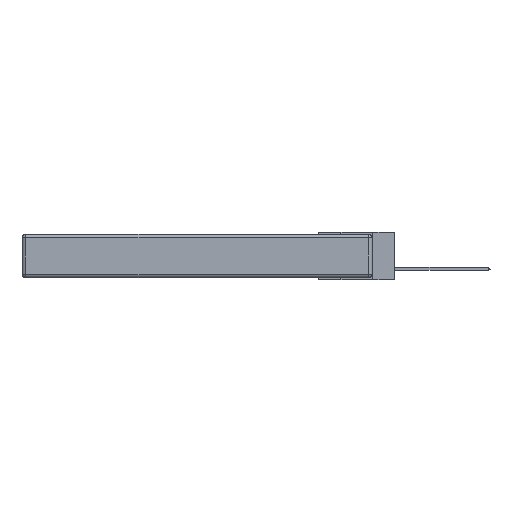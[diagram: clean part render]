
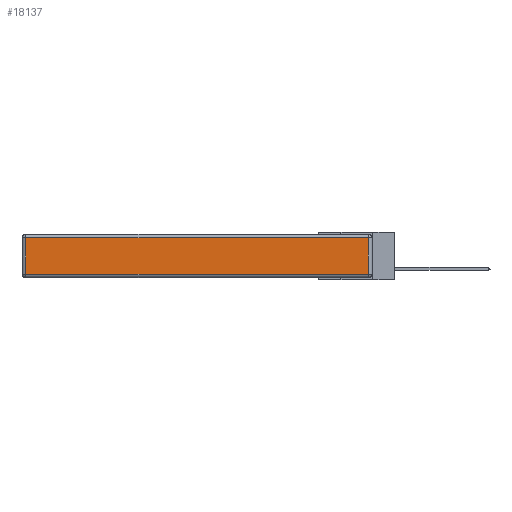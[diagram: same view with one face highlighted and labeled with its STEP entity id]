
A CAD part, left-side view. The second image highlights one B-rep face of the part: STEP entity #18137.
In plain terms, the highlighted planar face has unit normal (-1, 0, 0).
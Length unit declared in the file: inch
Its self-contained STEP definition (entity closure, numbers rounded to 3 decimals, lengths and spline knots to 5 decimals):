
#7 = DIRECTION ( 'NONE',  ( -1., 0., 0. ) ) ;
#1589 = CARTESIAN_POINT ( 'NONE',  ( 0., 2.72, -0.03 ) ) ;
#1965 = CARTESIAN_POINT ( 'NONE',  ( 0., 0.03, -0.343 ) ) ;
#2236 = CARTESIAN_POINT ( 'NONE',  ( 0., 0., -0.343 ) ) ;
#4499 = ORIENTED_EDGE ( 'NONE', *, *, #5396, .T. ) ;
#4649 = EDGE_LOOP ( 'NONE', ( #9485, #4499, #24535, #13601 ) ) ;
#5396 = EDGE_CURVE ( 'NONE', #16382, #19839, #21255, .T. ) ;
#5569 = DIRECTION ( 'NONE',  ( 0., 0., -1. ) ) ;
#6389 = AXIS2_PLACEMENT_3D ( 'NONE', #2236, #7, #12685 ) ;
#6978 = EDGE_CURVE ( 'NONE', #19839, #25002, #9342, .T. ) ;
#8350 = VECTOR ( 'NONE', #25428, 39.37008 ) ;
#8665 = DIRECTION ( 'NONE',  ( 0., 1., 0. ) ) ;
#9079 = LINE ( 'NONE', #18195, #26648 ) ;
#9342 = LINE ( 'NONE', #13171, #26913 ) ;
#9485 = ORIENTED_EDGE ( 'NONE', *, *, #14847, .T. ) ;
#12685 = DIRECTION ( 'NONE',  ( 0., 0., 1. ) ) ;
#13171 = CARTESIAN_POINT ( 'NONE',  ( 0., 2.75, -0.03 ) ) ;
#13601 = ORIENTED_EDGE ( 'NONE', *, *, #20556, .T. ) ;
#14847 = EDGE_CURVE ( 'NONE', #24654, #16382, #23490, .T. ) ;
#16382 = VERTEX_POINT ( 'NONE', #22212 ) ;
#17675 = CARTESIAN_POINT ( 'NONE',  ( 0., 0.03, -0.03 ) ) ;
#18137 = ADVANCED_FACE ( 'NONE', ( #20768 ), #25420, .T. ) ;
#18195 = CARTESIAN_POINT ( 'NONE',  ( 0., 2.72, -0.343 ) ) ;
#18600 = CARTESIAN_POINT ( 'NONE',  ( 0., 0., -0.313 ) ) ;
#19839 = VERTEX_POINT ( 'NONE', #17675 ) ;
#20556 = EDGE_CURVE ( 'NONE', #25002, #24654, #9079, .T. ) ;
#20768 = FACE_OUTER_BOUND ( 'NONE', #4649, .T. ) ;
#20805 = DIRECTION ( 'NONE',  ( 0., -1., 0. ) ) ;
#21255 = LINE ( 'NONE', #1965, #8350 ) ;
#22212 = CARTESIAN_POINT ( 'NONE',  ( 0., 0.03, -0.313 ) ) ;
#23490 = LINE ( 'NONE', #18600, #27153 ) ;
#23760 = CARTESIAN_POINT ( 'NONE',  ( 0., 2.72, -0.313 ) ) ;
#24535 = ORIENTED_EDGE ( 'NONE', *, *, #6978, .T. ) ;
#24654 = VERTEX_POINT ( 'NONE', #23760 ) ;
#25002 = VERTEX_POINT ( 'NONE', #1589 ) ;
#25420 = PLANE ( 'NONE',  #6389 ) ;
#25428 = DIRECTION ( 'NONE',  ( 0., 0., 1. ) ) ;
#26648 = VECTOR ( 'NONE', #5569, 39.37008 ) ;
#26913 = VECTOR ( 'NONE', #8665, 39.37008 ) ;
#27153 = VECTOR ( 'NONE', #20805, 39.37008 ) ;
